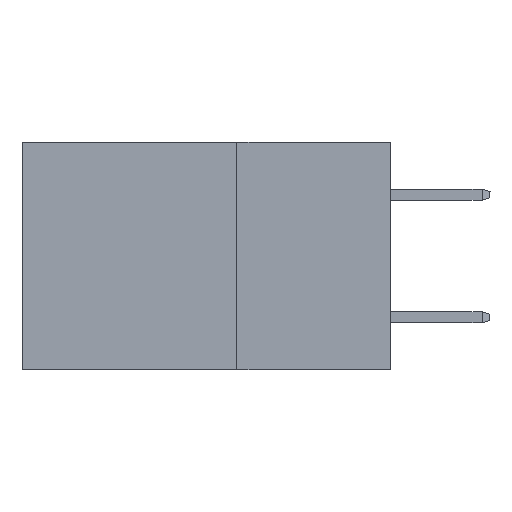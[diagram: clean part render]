
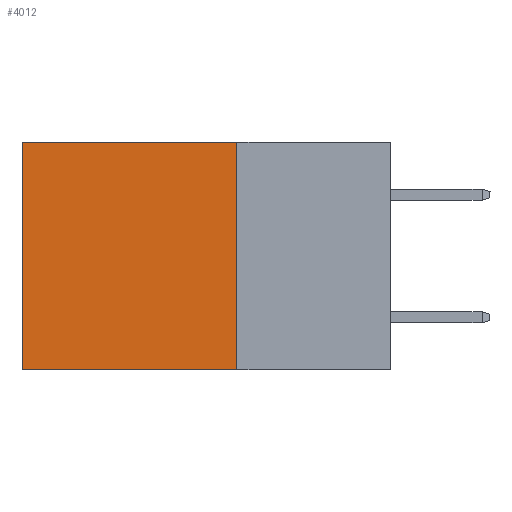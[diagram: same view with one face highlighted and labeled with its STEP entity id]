
A CAD part, left-side view. The second image highlights one B-rep face of the part: STEP entity #4012.
In plain terms, the highlighted planar face has unit normal (-1, 0, 0).
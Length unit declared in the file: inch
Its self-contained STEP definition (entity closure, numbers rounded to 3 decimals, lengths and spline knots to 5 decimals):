
#1001 = VECTOR ( 'NONE', #15173, 39.37008 ) ;
#1219 = AXIS2_PLACEMENT_3D ( 'NONE', #14325, #6593, #17455 ) ;
#1959 = CARTESIAN_POINT ( 'NONE',  ( 0.2875, 0.6, 0. ) ) ;
#2133 = VERTEX_POINT ( 'NONE', #3597 ) ;
#2490 = VECTOR ( 'NONE', #14100, 39.37008 ) ;
#3168 = CARTESIAN_POINT ( 'NONE',  ( 0.2875, 0.25, 0. ) ) ;
#3597 = CARTESIAN_POINT ( 'NONE',  ( 0.2875, 0.6, -0.37 ) ) ;
#4012 = ADVANCED_FACE ( 'NONE', ( #17457 ), #14393, .F. ) ;
#4817 = ORIENTED_EDGE ( 'NONE', *, *, #15174, .F. ) ;
#4884 = CARTESIAN_POINT ( 'NONE',  ( 0.2875, 0.25, 0. ) ) ;
#5821 = LINE ( 'NONE', #4884, #17733 ) ;
#6593 = DIRECTION ( 'NONE',  ( 1., 0., 0. ) ) ;
#6913 = LINE ( 'NONE', #11048, #2490 ) ;
#8045 = VERTEX_POINT ( 'NONE', #1959 ) ;
#8201 = ORIENTED_EDGE ( 'NONE', *, *, #12059, .T. ) ;
#9933 = DIRECTION ( 'NONE',  ( 0., 0., -1. ) ) ;
#11048 = CARTESIAN_POINT ( 'NONE',  ( 0.2875, 0.25, -0.37 ) ) ;
#11383 = CARTESIAN_POINT ( 'NONE',  ( 0.2875, 0.25, -0.37 ) ) ;
#12059 = EDGE_CURVE ( 'NONE', #18642, #8045, #5821, .T. ) ;
#12151 = CARTESIAN_POINT ( 'NONE',  ( 0.2875, 0.25, 0. ) ) ;
#12803 = DIRECTION ( 'NONE',  ( 0., 1., 0. ) ) ;
#13073 = CARTESIAN_POINT ( 'NONE',  ( 0.2875, 0.6, 0. ) ) ;
#13149 = EDGE_CURVE ( 'NONE', #18642, #19851, #17935, .T. ) ;
#13465 = ORIENTED_EDGE ( 'NONE', *, *, #13149, .F. ) ;
#13892 = LINE ( 'NONE', #13073, #17936 ) ;
#14100 = DIRECTION ( 'NONE',  ( 0., 1., 0. ) ) ;
#14325 = CARTESIAN_POINT ( 'NONE',  ( 0.2875, 0.25, 0. ) ) ;
#14393 = PLANE ( 'NONE',  #1219 ) ;
#15107 = ORIENTED_EDGE ( 'NONE', *, *, #19911, .T. ) ;
#15173 = DIRECTION ( 'NONE',  ( 0., 0., -1. ) ) ;
#15174 = EDGE_CURVE ( 'NONE', #19851, #2133, #6913, .T. ) ;
#17455 = DIRECTION ( 'NONE',  ( 0., 0., -1. ) ) ;
#17457 = FACE_OUTER_BOUND ( 'NONE', #17725, .T. ) ;
#17725 = EDGE_LOOP ( 'NONE', ( #15107, #4817, #13465, #8201 ) ) ;
#17733 = VECTOR ( 'NONE', #12803, 39.37008 ) ;
#17935 = LINE ( 'NONE', #12151, #1001 ) ;
#17936 = VECTOR ( 'NONE', #9933, 39.37008 ) ;
#18642 = VERTEX_POINT ( 'NONE', #3168 ) ;
#19851 = VERTEX_POINT ( 'NONE', #11383 ) ;
#19911 = EDGE_CURVE ( 'NONE', #8045, #2133, #13892, .T. ) ;
